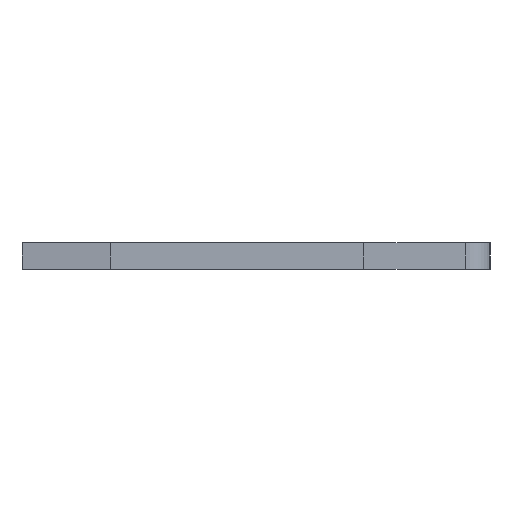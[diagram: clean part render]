
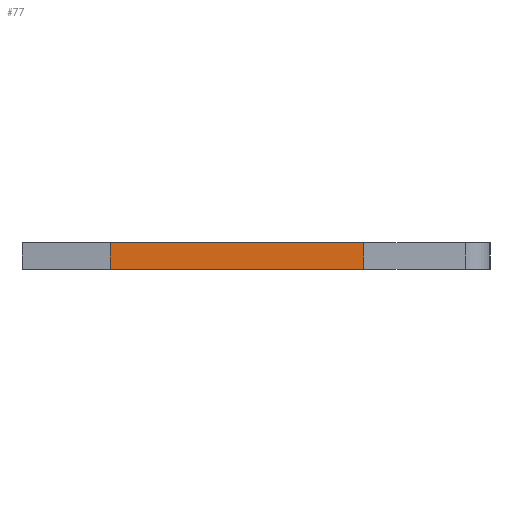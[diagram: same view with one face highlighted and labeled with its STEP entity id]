
A CAD part, left-side view. The second image highlights one B-rep face of the part: STEP entity #77.
In plain terms, the highlighted face is planar.
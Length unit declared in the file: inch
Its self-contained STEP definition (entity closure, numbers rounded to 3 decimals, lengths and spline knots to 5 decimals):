
#14 = ORIENTED_EDGE ( 'NONE', *, *, #895, .T. ) ;
#43 = VECTOR ( 'NONE', #958, 39.37008 ) ;
#77 = ADVANCED_FACE ( 'NONE', ( #839 ), #1276, .F. ) ;
#99 = VECTOR ( 'NONE', #464, 39.37008 ) ;
#146 = EDGE_CURVE ( 'NONE', #529, #802, #1144, .T. ) ;
#162 = CARTESIAN_POINT ( 'NONE',  ( 0.013, -0.099, -0.0575 ) ) ;
#245 = CARTESIAN_POINT ( 'NONE',  ( -0.013, 0.146, -0.0575 ) ) ;
#268 = LINE ( 'NONE', #162, #565 ) ;
#314 = CARTESIAN_POINT ( 'NONE',  ( 0.013, 0.146, -0.0575 ) ) ;
#357 = LINE ( 'NONE', #1423, #43 ) ;
#361 = DIRECTION ( 'NONE',  ( 0., 1., 0. ) ) ;
#381 = AXIS2_PLACEMENT_3D ( 'NONE', #1024, #444, #664 ) ;
#436 = VERTEX_POINT ( 'NONE', #806 ) ;
#444 = DIRECTION ( 'NONE',  ( 0., 0., 1. ) ) ;
#451 = CARTESIAN_POINT ( 'NONE',  ( 0.013, -0.099, -0.0575 ) ) ;
#464 = DIRECTION ( 'NONE',  ( -1., 0., 0. ) ) ;
#502 = CARTESIAN_POINT ( 'NONE',  ( -0.013, 0.146, -0.0575 ) ) ;
#529 = VERTEX_POINT ( 'NONE', #849 ) ;
#565 = VECTOR ( 'NONE', #1113, 39.37008 ) ;
#570 = EDGE_CURVE ( 'NONE', #1165, #529, #357, .T. ) ;
#577 = EDGE_CURVE ( 'NONE', #436, #802, #993, .T. ) ;
#589 = ORIENTED_EDGE ( 'NONE', *, *, #570, .F. ) ;
#664 = DIRECTION ( 'NONE',  ( 1., 0., 0. ) ) ;
#672 = VECTOR ( 'NONE', #361, 39.37008 ) ;
#784 = ORIENTED_EDGE ( 'NONE', *, *, #577, .T. ) ;
#802 = VERTEX_POINT ( 'NONE', #502 ) ;
#806 = CARTESIAN_POINT ( 'NONE',  ( -0.013, -0.099, -0.0575 ) ) ;
#839 = FACE_OUTER_BOUND ( 'NONE', #1258, .T. ) ;
#849 = CARTESIAN_POINT ( 'NONE',  ( 0.013, 0.146, -0.0575 ) ) ;
#895 = EDGE_CURVE ( 'NONE', #1165, #436, #268, .T. ) ;
#958 = DIRECTION ( 'NONE',  ( 0., 1., 0. ) ) ;
#993 = LINE ( 'NONE', #245, #672 ) ;
#1024 = CARTESIAN_POINT ( 'NONE',  ( 0.013, 0.146, -0.0575 ) ) ;
#1113 = DIRECTION ( 'NONE',  ( -1., 0., 0. ) ) ;
#1144 = LINE ( 'NONE', #314, #99 ) ;
#1165 = VERTEX_POINT ( 'NONE', #451 ) ;
#1258 = EDGE_LOOP ( 'NONE', ( #784, #1303, #589, #14 ) ) ;
#1276 = PLANE ( 'NONE',  #381 ) ;
#1303 = ORIENTED_EDGE ( 'NONE', *, *, #146, .F. ) ;
#1423 = CARTESIAN_POINT ( 'NONE',  ( 0.013, 0.146, -0.0575 ) ) ;
